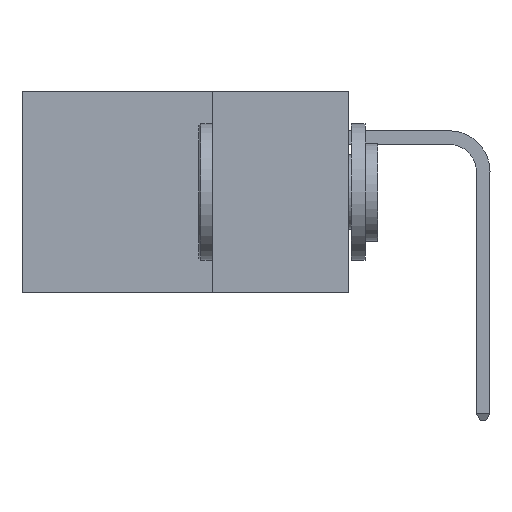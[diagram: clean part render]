
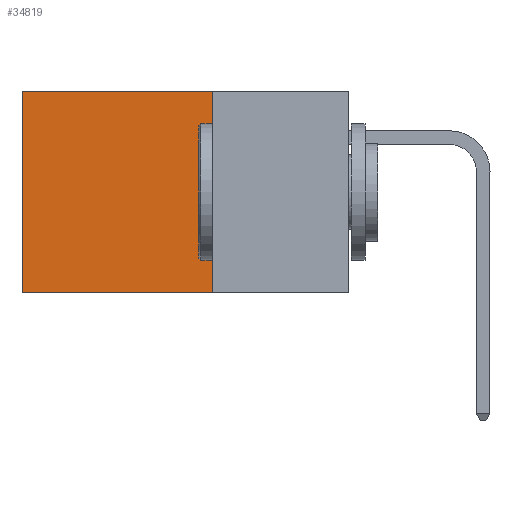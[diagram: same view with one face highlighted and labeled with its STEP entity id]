
A CAD part, left-side view. The second image highlights one B-rep face of the part: STEP entity #34819.
In plain terms, the highlighted planar face has unit normal (-1, 0, 0).
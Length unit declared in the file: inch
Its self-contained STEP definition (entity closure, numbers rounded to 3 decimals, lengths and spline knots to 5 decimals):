
#421 = DIRECTION ( 'NONE',  ( 0., 1., 0. ) ) ;
#744 = DIRECTION ( 'NONE',  ( 0., 0., -1. ) ) ;
#2677 = ORIENTED_EDGE ( 'NONE', *, *, #12423, .F. ) ;
#5115 = CARTESIAN_POINT ( 'NONE',  ( 0.2875, 0.25, -0.37 ) ) ;
#6854 = PLANE ( 'NONE',  #12336 ) ;
#7971 = LINE ( 'NONE', #36276, #15062 ) ;
#9595 = VERTEX_POINT ( 'NONE', #33086 ) ;
#9871 = DIRECTION ( 'NONE',  ( 0., 0., -1. ) ) ;
#12336 = AXIS2_PLACEMENT_3D ( 'NONE', #12770, #28027, #9871 ) ;
#12423 = EDGE_CURVE ( 'NONE', #9595, #14846, #7971, .T. ) ;
#12770 = CARTESIAN_POINT ( 'NONE',  ( 0.2875, 0.25, 0. ) ) ;
#13368 = VERTEX_POINT ( 'NONE', #31256 ) ;
#13967 = EDGE_CURVE ( 'NONE', #13368, #39025, #25049, .T. ) ;
#14503 = EDGE_CURVE ( 'NONE', #9595, #13368, #21151, .T. ) ;
#14846 = VERTEX_POINT ( 'NONE', #5115 ) ;
#14960 = VECTOR ( 'NONE', #421, 39.37008 ) ;
#15062 = VECTOR ( 'NONE', #21294, 39.37008 ) ;
#15854 = ORIENTED_EDGE ( 'NONE', *, *, #14503, .T. ) ;
#16295 = CARTESIAN_POINT ( 'NONE',  ( 0.2875, 0.6, -0.37 ) ) ;
#17964 = ORIENTED_EDGE ( 'NONE', *, *, #34310, .F. ) ;
#20531 = LINE ( 'NONE', #31627, #26696 ) ;
#21151 = LINE ( 'NONE', #21675, #14960 ) ;
#21294 = DIRECTION ( 'NONE',  ( 0., 0., -1. ) ) ;
#21675 = CARTESIAN_POINT ( 'NONE',  ( 0.2875, 0.25, 0. ) ) ;
#22633 = ORIENTED_EDGE ( 'NONE', *, *, #13967, .T. ) ;
#23838 = FACE_OUTER_BOUND ( 'NONE', #28201, .T. ) ;
#25049 = LINE ( 'NONE', #28177, #32996 ) ;
#26696 = VECTOR ( 'NONE', #34617, 39.37008 ) ;
#28027 = DIRECTION ( 'NONE',  ( 1., 0., 0. ) ) ;
#28177 = CARTESIAN_POINT ( 'NONE',  ( 0.2875, 0.6, 0. ) ) ;
#28201 = EDGE_LOOP ( 'NONE', ( #22633, #17964, #2677, #15854 ) ) ;
#31256 = CARTESIAN_POINT ( 'NONE',  ( 0.2875, 0.6, 0. ) ) ;
#31627 = CARTESIAN_POINT ( 'NONE',  ( 0.2875, 0.25, -0.37 ) ) ;
#32996 = VECTOR ( 'NONE', #744, 39.37008 ) ;
#33086 = CARTESIAN_POINT ( 'NONE',  ( 0.2875, 0.25, 0. ) ) ;
#34310 = EDGE_CURVE ( 'NONE', #14846, #39025, #20531, .T. ) ;
#34617 = DIRECTION ( 'NONE',  ( 0., 1., 0. ) ) ;
#34819 = ADVANCED_FACE ( 'NONE', ( #23838 ), #6854, .F. ) ;
#36276 = CARTESIAN_POINT ( 'NONE',  ( 0.2875, 0.25, 0. ) ) ;
#39025 = VERTEX_POINT ( 'NONE', #16295 ) ;
